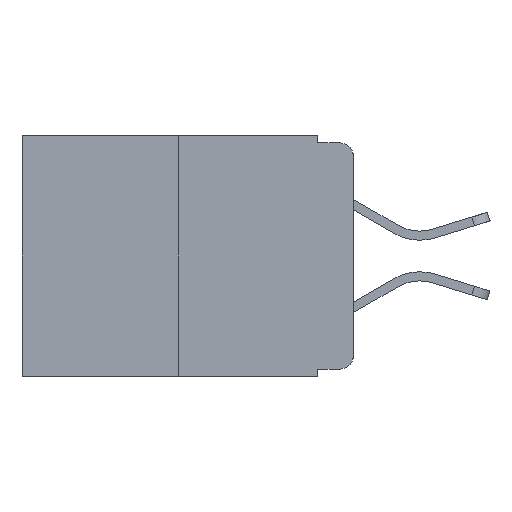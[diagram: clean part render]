
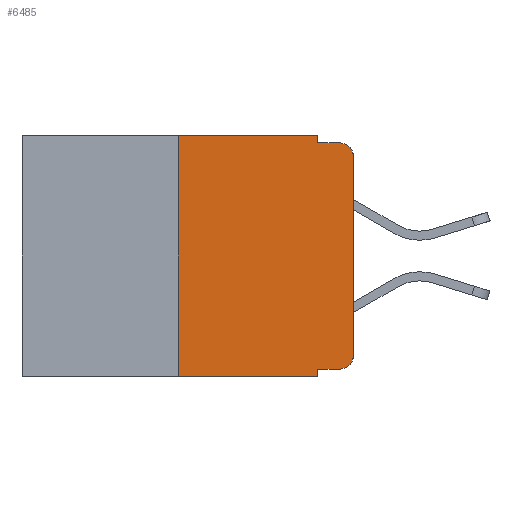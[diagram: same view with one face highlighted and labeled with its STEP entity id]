
A CAD part, left-side view. The second image highlights one B-rep face of the part: STEP entity #6485.
In plain terms, the highlighted planar face has unit normal (-1, 0, 0).
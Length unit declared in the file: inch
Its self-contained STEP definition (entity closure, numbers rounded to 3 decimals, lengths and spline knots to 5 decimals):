
#114 = DIRECTION ( 'NONE',  ( -1., 0., 0. ) ) ;
#134 = ORIENTED_EDGE ( 'NONE', *, *, #4026, .T. ) ;
#392 = VECTOR ( 'NONE', #4378, 39.37008 ) ;
#464 = ORIENTED_EDGE ( 'NONE', *, *, #6180, .F. ) ;
#590 = CARTESIAN_POINT ( 'NONE',  ( 0., 0., -0.03 ) ) ;
#628 = VERTEX_POINT ( 'NONE', #13028 ) ;
#683 = PLANE ( 'NONE',  #5225 ) ;
#780 = DIRECTION ( 'NONE',  ( 1., 0., 0. ) ) ;
#844 = CARTESIAN_POINT ( 'NONE',  ( 0., 0.02, -0.313 ) ) ;
#930 = FACE_OUTER_BOUND ( 'NONE', #11643, .T. ) ;
#1113 = CARTESIAN_POINT ( 'NONE',  ( 0., 0.473, 0. ) ) ;
#1643 = CARTESIAN_POINT ( 'NONE',  ( 0., 0.473, -0.343 ) ) ;
#1677 = CARTESIAN_POINT ( 'NONE',  ( 0., 0., 0. ) ) ;
#1741 = EDGE_CURVE ( 'NONE', #628, #5142, #2723, .T. ) ;
#1767 = ORIENTED_EDGE ( 'NONE', *, *, #11735, .T. ) ;
#1994 = DIRECTION ( 'NONE',  ( 0., 0., -1. ) ) ;
#2203 = EDGE_CURVE ( 'NONE', #7820, #3501, #2709, .T. ) ;
#2373 = DIRECTION ( 'NONE',  ( 0., -1., 0. ) ) ;
#2387 = LINE ( 'NONE', #1113, #7774 ) ;
#2600 = ORIENTED_EDGE ( 'NONE', *, *, #1741, .T. ) ;
#2709 = LINE ( 'NONE', #1643, #12487 ) ;
#2723 = LINE ( 'NONE', #1677, #12784 ) ;
#2851 = CIRCLE ( 'NONE', #5068, 0.02 ) ;
#3501 = VERTEX_POINT ( 'NONE', #7009 ) ;
#3534 = LINE ( 'NONE', #5784, #8687 ) ;
#3592 = CARTESIAN_POINT ( 'NONE',  ( 0., 0.051, -0.01 ) ) ;
#3637 = CARTESIAN_POINT ( 'NONE',  ( 0., 0.051, -0.333 ) ) ;
#3663 = CARTESIAN_POINT ( 'NONE',  ( 0., 0.051, 0. ) ) ;
#4026 = EDGE_CURVE ( 'NONE', #5142, #6847, #9359, .T. ) ;
#4067 = VERTEX_POINT ( 'NONE', #3637 ) ;
#4072 = ORIENTED_EDGE ( 'NONE', *, *, #5368, .F. ) ;
#4378 = DIRECTION ( 'NONE',  ( 0., -1., 0. ) ) ;
#4482 = CARTESIAN_POINT ( 'NONE',  ( 0., 0.25, 0. ) ) ;
#4574 = DIRECTION ( 'NONE',  ( 0., 0., 1. ) ) ;
#4589 = DIRECTION ( 'NONE',  ( 0., 0., -1. ) ) ;
#4968 = ORIENTED_EDGE ( 'NONE', *, *, #8168, .F. ) ;
#5068 = AXIS2_PLACEMENT_3D ( 'NONE', #844, #8340, #1994 ) ;
#5142 = VERTEX_POINT ( 'NONE', #590 ) ;
#5225 = AXIS2_PLACEMENT_3D ( 'NONE', #7372, #780, #8297 ) ;
#5279 = CARTESIAN_POINT ( 'NONE',  ( 0., 0.051, 0. ) ) ;
#5368 = EDGE_CURVE ( 'NONE', #10907, #9024, #2387, .T. ) ;
#5441 = ORIENTED_EDGE ( 'NONE', *, *, #10574, .F. ) ;
#5454 = LINE ( 'NONE', #5279, #12301 ) ;
#5784 = CARTESIAN_POINT ( 'NONE',  ( 0., 0.051, -0.333 ) ) ;
#6180 = EDGE_CURVE ( 'NONE', #8341, #6847, #8595, .T. ) ;
#6291 = VECTOR ( 'NONE', #6923, 39.37008 ) ;
#6485 = ADVANCED_FACE ( 'NONE', ( #930 ), #683, .F. ) ;
#6822 = CARTESIAN_POINT ( 'NONE',  ( 0., 0.02, -0.03 ) ) ;
#6847 = VERTEX_POINT ( 'NONE', #11016 ) ;
#6923 = DIRECTION ( 'NONE',  ( 0., 0., 1. ) ) ;
#7009 = CARTESIAN_POINT ( 'NONE',  ( 0., 0.051, -0.343 ) ) ;
#7123 = CARTESIAN_POINT ( 'NONE',  ( 0., 0.02, -0.333 ) ) ;
#7372 = CARTESIAN_POINT ( 'NONE',  ( 0., 0.473, 0. ) ) ;
#7618 = DIRECTION ( 'NONE',  ( 0., -1., 0. ) ) ;
#7774 = VECTOR ( 'NONE', #7618, 39.37008 ) ;
#7796 = DIRECTION ( 'NONE',  ( 0., 0., -1. ) ) ;
#7820 = VERTEX_POINT ( 'NONE', #10144 ) ;
#7904 = ORIENTED_EDGE ( 'NONE', *, *, #9995, .F. ) ;
#8168 = EDGE_CURVE ( 'NONE', #9024, #8341, #8864, .T. ) ;
#8297 = DIRECTION ( 'NONE',  ( 0., 0., -1. ) ) ;
#8340 = DIRECTION ( 'NONE',  ( -1., 0., 0. ) ) ;
#8341 = VERTEX_POINT ( 'NONE', #3592 ) ;
#8595 = LINE ( 'NONE', #10242, #392 ) ;
#8687 = VECTOR ( 'NONE', #9662, 39.37008 ) ;
#8731 = VERTEX_POINT ( 'NONE', #7123 ) ;
#8864 = LINE ( 'NONE', #11256, #10932 ) ;
#9024 = VERTEX_POINT ( 'NONE', #3663 ) ;
#9230 = ORIENTED_EDGE ( 'NONE', *, *, #11146, .T. ) ;
#9359 = CIRCLE ( 'NONE', #10919, 0.02 ) ;
#9662 = DIRECTION ( 'NONE',  ( 0., -1., 0. ) ) ;
#9995 = EDGE_CURVE ( 'NONE', #7820, #10907, #11192, .T. ) ;
#10144 = CARTESIAN_POINT ( 'NONE',  ( 0., 0.25, -0.343 ) ) ;
#10242 = CARTESIAN_POINT ( 'NONE',  ( 0., 0.051, -0.01 ) ) ;
#10553 = CARTESIAN_POINT ( 'NONE',  ( 0., 0.25, 0. ) ) ;
#10574 = EDGE_CURVE ( 'NONE', #4067, #3501, #5454, .T. ) ;
#10907 = VERTEX_POINT ( 'NONE', #4482 ) ;
#10919 = AXIS2_PLACEMENT_3D ( 'NONE', #6822, #114, #7796 ) ;
#10932 = VECTOR ( 'NONE', #4589, 39.37008 ) ;
#11016 = CARTESIAN_POINT ( 'NONE',  ( 0., 0.02, -0.01 ) ) ;
#11146 = EDGE_CURVE ( 'NONE', #4067, #8731, #3534, .T. ) ;
#11192 = LINE ( 'NONE', #10553, #6291 ) ;
#11256 = CARTESIAN_POINT ( 'NONE',  ( 0., 0.051, 0. ) ) ;
#11643 = EDGE_LOOP ( 'NONE', ( #2600, #134, #464, #4968, #4072, #7904, #11943, #5441, #9230, #1767 ) ) ;
#11735 = EDGE_CURVE ( 'NONE', #8731, #628, #2851, .T. ) ;
#11943 = ORIENTED_EDGE ( 'NONE', *, *, #2203, .T. ) ;
#12301 = VECTOR ( 'NONE', #12759, 39.37008 ) ;
#12487 = VECTOR ( 'NONE', #2373, 39.37008 ) ;
#12759 = DIRECTION ( 'NONE',  ( 0., 0., -1. ) ) ;
#12784 = VECTOR ( 'NONE', #4574, 39.37008 ) ;
#13028 = CARTESIAN_POINT ( 'NONE',  ( 0., 0., -0.313 ) ) ;
